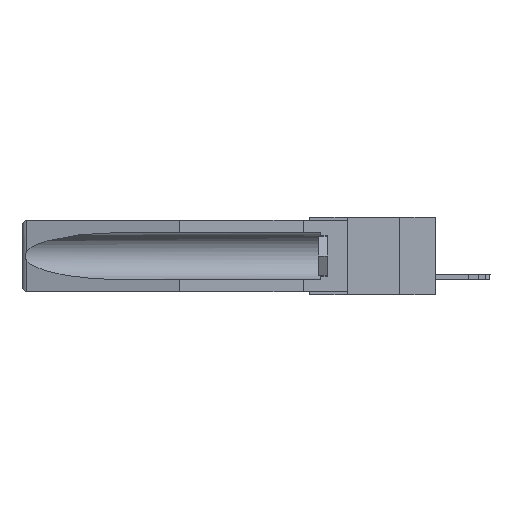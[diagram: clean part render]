
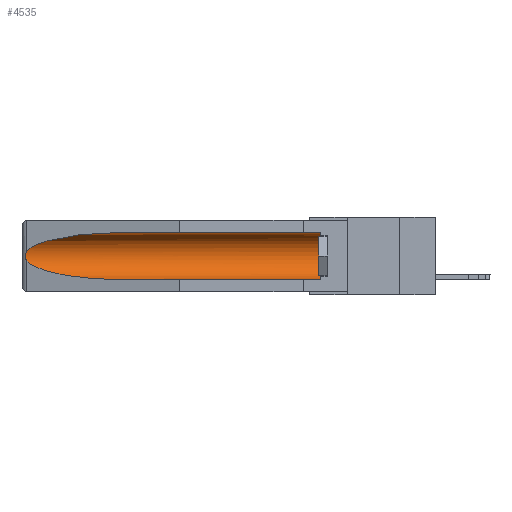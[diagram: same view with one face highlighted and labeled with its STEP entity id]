
A CAD part, left-side view. The second image highlights one B-rep face of the part: STEP entity #4535.
In plain terms, the highlighted cylindrical face has radius 2.857 mm (diameter 5.715 mm), a partial arc.
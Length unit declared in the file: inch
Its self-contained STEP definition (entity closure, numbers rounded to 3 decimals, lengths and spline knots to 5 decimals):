
#23 = VECTOR ( 'NONE', #1970, 39.37008 ) ;
#238 = EDGE_CURVE ( 'NONE', #14023, #22714, #4664, .T. ) ;
#608 = CARTESIAN_POINT ( 'NONE',  ( 0.155, 1.07973, -0.284 ) ) ;
#1061 = VERTEX_POINT ( 'NONE', #1359 ) ;
#1359 = CARTESIAN_POINT ( 'NONE',  ( 0.155, 0.126, -0.059 ) ) ;
#1443 = CARTESIAN_POINT ( 'NONE',  ( 0.155, 1.07973, -0.284 ) ) ;
#1750 = DIRECTION ( 'NONE',  ( 0., -1., 0. ) ) ;
#1923 = CARTESIAN_POINT ( 'NONE',  ( 0.26654, 1.53092, -0.15636 ) ) ;
#1970 = DIRECTION ( 'NONE',  ( 0., 1., 0. ) ) ;
#2396 = ORIENTED_EDGE ( 'NONE', *, *, #14264, .F. ) ;
#2642 = CARTESIAN_POINT ( 'NONE',  ( 0.26537, 1.52718, -0.19328 ) ) ;
#3341 = CARTESIAN_POINT ( 'NONE',  ( 0.155, 1.07973, -0.059 ) ) ;
#3805 = CARTESIAN_POINT ( 'NONE',  ( 0.2673, 1.53269, -0.17917 ) ) ;
#3877 = CARTESIAN_POINT ( 'NONE',  ( 0.2675, 1.53308, -0.16763 ) ) ;
#4098 = EDGE_CURVE ( 'NONE', #16130, #1061, #23097, .T. ) ;
#4483 = CYLINDRICAL_SURFACE ( 'NONE', #20495, 0.1125 ) ;
#4535 = ADVANCED_FACE ( 'NONE', ( #17682 ), #4483, .F. ) ;
#4664 =( BOUNDED_CURVE ( )  B_SPLINE_CURVE ( 3, ( #3341, #19513, #7099, #5149 ),
 .UNSPECIFIED., .F., .T. ) 
 B_SPLINE_CURVE_WITH_KNOTS ( ( 4, 4 ),
 ( 4.71239, 6.08839 ),
 .UNSPECIFIED. ) 
 CURVE ( )  GEOMETRIC_REPRESENTATION_ITEM ( )  RATIONAL_B_SPLINE_CURVE ( ( 1., 0.848, 0.848, 1. ) ) 
 REPRESENTATION_ITEM ( '' )  );
#4702 = CARTESIAN_POINT ( 'NONE',  ( 0.155, 0.126, -0.284 ) ) ;
#5149 = CARTESIAN_POINT ( 'NONE',  ( 0.26537, 1.52718, -0.14972 ) ) ;
#5423 = CARTESIAN_POINT ( 'NONE',  ( 0.155, 0.126, -0.1715 ) ) ;
#6719 = EDGE_CURVE ( 'NONE', #16333, #20878, #18942, .T. ) ;
#6882 = ORIENTED_EDGE ( 'NONE', *, *, #10730, .T. ) ;
#7099 = CARTESIAN_POINT ( 'NONE',  ( 0.25451, 1.48313, -0.09465 ) ) ;
#7341 = CARTESIAN_POINT ( 'NONE',  ( 0.26597, 1.52961, -0.15275 ) ) ;
#7430 = CARTESIAN_POINT ( 'NONE',  ( 0.26655, 1.53094, -0.18657 ) ) ;
#7518 = CARTESIAN_POINT ( 'NONE',  ( 0.155, -0.30754, -0.284 ) ) ;
#7916 = LINE ( 'NONE', #19800, #23 ) ;
#7919 = CARTESIAN_POINT ( 'NONE',  ( 0.25451, 1.48313, -0.24835 ) ) ;
#8495 = CARTESIAN_POINT ( 'NONE',  ( 0.26537, 1.52718, -0.14972 ) ) ;
#8575 = B_SPLINE_CURVE_WITH_KNOTS ( 'NONE', 3,
 ( #12681, #7341, #1923, #19912, #3877, #21747, #3805, #7430, #9222, #22064 ),
 .UNSPECIFIED., .F., .F.,
 ( 4, 2, 2, 2, 4 ),
 ( 0., 0.00029, 0.00058, 0.00087, 0.00117 ),
 .UNSPECIFIED. ) ;
#8822 = CARTESIAN_POINT ( 'NONE',  ( 0.155, 1.07973, -0.059 ) ) ;
#9222 = CARTESIAN_POINT ( 'NONE',  ( 0.26597, 1.5296, -0.19026 ) ) ;
#9309 = EDGE_LOOP ( 'NONE', ( #12797, #6882, #17016, #2396, #19611, #18860 ) ) ;
#10445 = DIRECTION ( 'NONE',  ( 0., 0., 1. ) ) ;
#10730 = EDGE_CURVE ( 'NONE', #22714, #16333, #8575, .T. ) ;
#10766 = CARTESIAN_POINT ( 'NONE',  ( 0.26537, 1.52718, -0.19328 ) ) ;
#12681 = CARTESIAN_POINT ( 'NONE',  ( 0.26537, 1.52718, -0.14972 ) ) ;
#12797 = ORIENTED_EDGE ( 'NONE', *, *, #238, .T. ) ;
#14023 = VERTEX_POINT ( 'NONE', #8822 ) ;
#14172 = LINE ( 'NONE', #7518, #17836 ) ;
#14264 = EDGE_CURVE ( 'NONE', #16130, #20878, #14172, .T. ) ;
#15852 = CARTESIAN_POINT ( 'NONE',  ( 0.155, -0.30754, -0.1715 ) ) ;
#16130 = VERTEX_POINT ( 'NONE', #4702 ) ;
#16333 = VERTEX_POINT ( 'NONE', #10766 ) ;
#16379 = EDGE_CURVE ( 'NONE', #1061, #14023, #7916, .T. ) ;
#16696 = DIRECTION ( 'NONE',  ( 0., 1., 0. ) ) ;
#17016 = ORIENTED_EDGE ( 'NONE', *, *, #6719, .T. ) ;
#17078 = CARTESIAN_POINT ( 'NONE',  ( 0.21114, 1.30732, -0.284 ) ) ;
#17494 = DIRECTION ( 'NONE',  ( 0., 1., 0. ) ) ;
#17682 = FACE_OUTER_BOUND ( 'NONE', #9309, .T. ) ;
#17836 = VECTOR ( 'NONE', #16696, 39.37008 ) ;
#18065 = DIRECTION ( 'NONE',  ( 0., 0., 1. ) ) ;
#18860 = ORIENTED_EDGE ( 'NONE', *, *, #16379, .T. ) ;
#18942 =( BOUNDED_CURVE ( )  B_SPLINE_CURVE ( 3, ( #2642, #7919, #17078, #608 ),
 .UNSPECIFIED., .F., .F. ) 
 B_SPLINE_CURVE_WITH_KNOTS ( ( 4, 4 ),
 ( 0.1948, 1.5708 ),
 .UNSPECIFIED. ) 
 CURVE ( )  GEOMETRIC_REPRESENTATION_ITEM ( )  RATIONAL_B_SPLINE_CURVE ( ( 1., 0.848, 0.848, 1. ) ) 
 REPRESENTATION_ITEM ( '' )  );
#19513 = CARTESIAN_POINT ( 'NONE',  ( 0.21114, 1.30732, -0.059 ) ) ;
#19611 = ORIENTED_EDGE ( 'NONE', *, *, #4098, .T. ) ;
#19800 = CARTESIAN_POINT ( 'NONE',  ( 0.155, -0.30754, -0.059 ) ) ;
#19912 = CARTESIAN_POINT ( 'NONE',  ( 0.2673, 1.5327, -0.16383 ) ) ;
#20495 = AXIS2_PLACEMENT_3D ( 'NONE', #15852, #17494, #10445 ) ;
#20632 = AXIS2_PLACEMENT_3D ( 'NONE', #5423, #1750, #18065 ) ;
#20878 = VERTEX_POINT ( 'NONE', #1443 ) ;
#21747 = CARTESIAN_POINT ( 'NONE',  ( 0.2675, 1.53308, -0.17534 ) ) ;
#22064 = CARTESIAN_POINT ( 'NONE',  ( 0.26537, 1.52718, -0.19328 ) ) ;
#22714 = VERTEX_POINT ( 'NONE', #8495 ) ;
#23097 = CIRCLE ( 'NONE', #20632, 0.1125 ) ;
